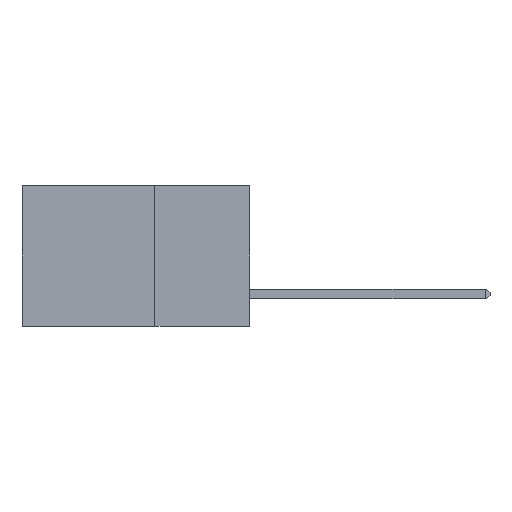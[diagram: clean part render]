
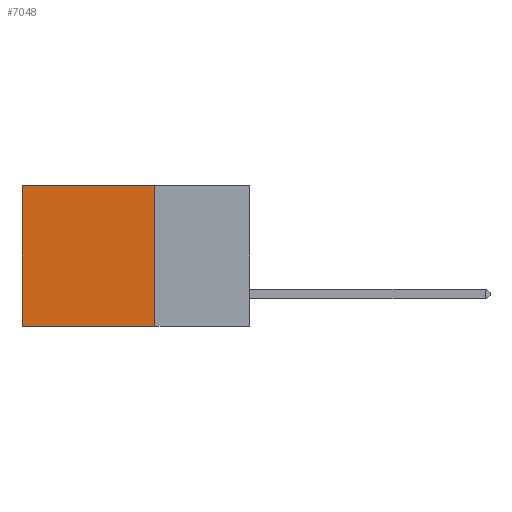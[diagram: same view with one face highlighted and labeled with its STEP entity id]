
A CAD part, left-side view. The second image highlights one B-rep face of the part: STEP entity #7048.
In plain terms, the highlighted planar face has unit normal (-1, 0, 0).
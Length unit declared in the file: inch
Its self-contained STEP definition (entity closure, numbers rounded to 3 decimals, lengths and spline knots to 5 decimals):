
#14 = CARTESIAN_POINT ( 'NONE',  ( 0.2875, 0.25, 0. ) ) ;
#295 = EDGE_CURVE ( 'NONE', #4132, #2464, #5730, .T. ) ;
#448 = CARTESIAN_POINT ( 'NONE',  ( 0.2875, 0.25, 0. ) ) ;
#476 = VECTOR ( 'NONE', #7189, 39.37008 ) ;
#928 = ORIENTED_EDGE ( 'NONE', *, *, #295, .F. ) ;
#942 = ORIENTED_EDGE ( 'NONE', *, *, #8895, .F. ) ;
#953 = DIRECTION ( 'NONE',  ( 0., 1., 0. ) ) ;
#1382 = CARTESIAN_POINT ( 'NONE',  ( 0.2875, 0.6, 0. ) ) ;
#1391 = ORIENTED_EDGE ( 'NONE', *, *, #8488, .T. ) ;
#1641 = VERTEX_POINT ( 'NONE', #1382 ) ;
#1677 = DIRECTION ( 'NONE',  ( 1., 0., 0. ) ) ;
#1823 = CARTESIAN_POINT ( 'NONE',  ( 0.2875, 0.25, 0. ) ) ;
#2427 = VECTOR ( 'NONE', #953, 39.37008 ) ;
#2464 = VERTEX_POINT ( 'NONE', #8040 ) ;
#3405 = EDGE_CURVE ( 'NONE', #1641, #5956, #8196, .T. ) ;
#3571 = DIRECTION ( 'NONE',  ( 0., 1., 0. ) ) ;
#3678 = DIRECTION ( 'NONE',  ( 0., 0., -1. ) ) ;
#3948 = AXIS2_PLACEMENT_3D ( 'NONE', #7470, #1677, #8444 ) ;
#4132 = VERTEX_POINT ( 'NONE', #448 ) ;
#5043 = LINE ( 'NONE', #14, #2427 ) ;
#5465 = CARTESIAN_POINT ( 'NONE',  ( 0.2875, 0.25, -0.37 ) ) ;
#5730 = LINE ( 'NONE', #1823, #8246 ) ;
#5956 = VERTEX_POINT ( 'NONE', #8795 ) ;
#7048 = ADVANCED_FACE ( 'NONE', ( #12144 ), #12013, .F. ) ;
#7189 = DIRECTION ( 'NONE',  ( 0., 0., -1. ) ) ;
#7401 = EDGE_LOOP ( 'NONE', ( #12024, #942, #928, #1391 ) ) ;
#7470 = CARTESIAN_POINT ( 'NONE',  ( 0.2875, 0.25, 0. ) ) ;
#7857 = VECTOR ( 'NONE', #3571, 39.37008 ) ;
#8040 = CARTESIAN_POINT ( 'NONE',  ( 0.2875, 0.25, -0.37 ) ) ;
#8118 = CARTESIAN_POINT ( 'NONE',  ( 0.2875, 0.6, 0. ) ) ;
#8196 = LINE ( 'NONE', #8118, #476 ) ;
#8246 = VECTOR ( 'NONE', #3678, 39.37008 ) ;
#8444 = DIRECTION ( 'NONE',  ( 0., 0., -1. ) ) ;
#8488 = EDGE_CURVE ( 'NONE', #4132, #1641, #5043, .T. ) ;
#8795 = CARTESIAN_POINT ( 'NONE',  ( 0.2875, 0.6, -0.37 ) ) ;
#8895 = EDGE_CURVE ( 'NONE', #2464, #5956, #10246, .T. ) ;
#10246 = LINE ( 'NONE', #5465, #7857 ) ;
#12013 = PLANE ( 'NONE',  #3948 ) ;
#12024 = ORIENTED_EDGE ( 'NONE', *, *, #3405, .T. ) ;
#12144 = FACE_OUTER_BOUND ( 'NONE', #7401, .T. ) ;
